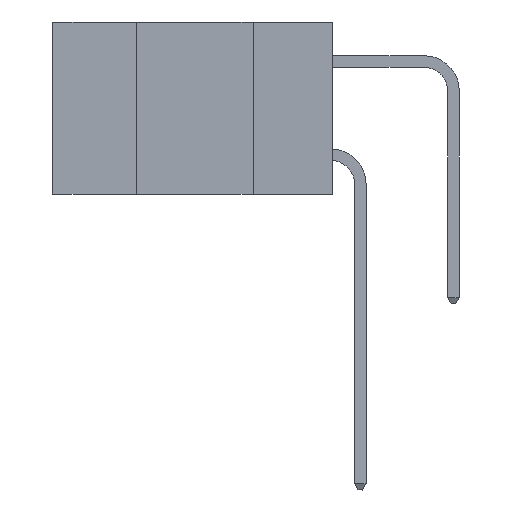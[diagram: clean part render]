
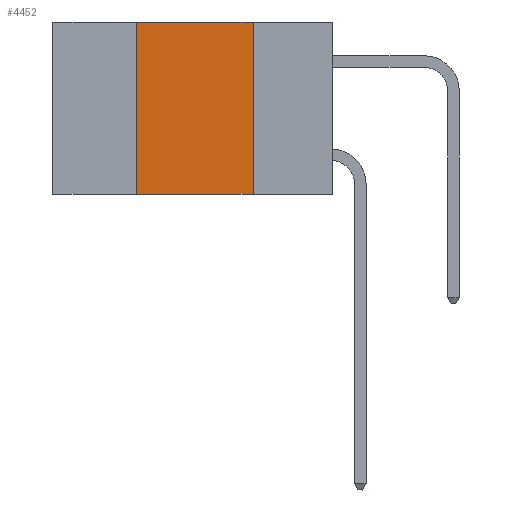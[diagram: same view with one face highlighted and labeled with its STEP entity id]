
A CAD part, left-side view. The second image highlights one B-rep face of the part: STEP entity #4452.
In plain terms, the highlighted planar face has unit normal (-1, 0, 0).
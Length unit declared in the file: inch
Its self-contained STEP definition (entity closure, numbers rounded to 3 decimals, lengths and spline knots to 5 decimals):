
#613 = ORIENTED_EDGE ( 'NONE', *, *, #7408, .F. ) ;
#865 = EDGE_CURVE ( 'NONE', #3802, #6660, #3411, .T. ) ;
#1081 = CARTESIAN_POINT ( 'NONE',  ( 0., 0.17, 0. ) ) ;
#1353 = EDGE_CURVE ( 'NONE', #3802, #3202, #12285, .T. ) ;
#3123 = CARTESIAN_POINT ( 'NONE',  ( 0., 0.17, 0. ) ) ;
#3202 = VERTEX_POINT ( 'NONE', #10478 ) ;
#3292 = DIRECTION ( 'NONE',  ( 0., 0., -1. ) ) ;
#3313 = CARTESIAN_POINT ( 'NONE',  ( 0., 0.42, -0.37 ) ) ;
#3347 = LINE ( 'NONE', #3123, #8274 ) ;
#3411 = LINE ( 'NONE', #4170, #5818 ) ;
#3802 = VERTEX_POINT ( 'NONE', #3313 ) ;
#3940 = EDGE_LOOP ( 'NONE', ( #7589, #613, #5367, #10637 ) ) ;
#4170 = CARTESIAN_POINT ( 'NONE',  ( 0., 0.42, 0. ) ) ;
#4452 = ADVANCED_FACE ( 'NONE', ( #8810 ), #8190, .F. ) ;
#4795 = CARTESIAN_POINT ( 'NONE',  ( 0., 0.6, 0. ) ) ;
#5168 = VECTOR ( 'NONE', #8775, 39.37008 ) ;
#5326 = CARTESIAN_POINT ( 'NONE',  ( 0., 0.6, 0. ) ) ;
#5367 = ORIENTED_EDGE ( 'NONE', *, *, #865, .F. ) ;
#5818 = VECTOR ( 'NONE', #9467, 39.37008 ) ;
#6283 = VECTOR ( 'NONE', #10449, 39.37008 ) ;
#6487 = CARTESIAN_POINT ( 'NONE',  ( 0., 0.6, -0.37 ) ) ;
#6660 = VERTEX_POINT ( 'NONE', #7673 ) ;
#6914 = VERTEX_POINT ( 'NONE', #1081 ) ;
#7408 = EDGE_CURVE ( 'NONE', #6660, #6914, #8781, .T. ) ;
#7589 = ORIENTED_EDGE ( 'NONE', *, *, #9722, .F. ) ;
#7673 = CARTESIAN_POINT ( 'NONE',  ( 0., 0.42, 0. ) ) ;
#8190 = PLANE ( 'NONE',  #11298 ) ;
#8274 = VECTOR ( 'NONE', #10811, 39.37008 ) ;
#8775 = DIRECTION ( 'NONE',  ( 0., -1., 0. ) ) ;
#8781 = LINE ( 'NONE', #4795, #6283 ) ;
#8810 = FACE_OUTER_BOUND ( 'NONE', #3940, .T. ) ;
#9137 = DIRECTION ( 'NONE',  ( 1., 0., 0. ) ) ;
#9467 = DIRECTION ( 'NONE',  ( 0., 0., 1. ) ) ;
#9722 = EDGE_CURVE ( 'NONE', #6914, #3202, #3347, .T. ) ;
#10449 = DIRECTION ( 'NONE',  ( 0., -1., 0. ) ) ;
#10478 = CARTESIAN_POINT ( 'NONE',  ( 0., 0.17, -0.37 ) ) ;
#10637 = ORIENTED_EDGE ( 'NONE', *, *, #1353, .T. ) ;
#10811 = DIRECTION ( 'NONE',  ( 0., 0., -1. ) ) ;
#11298 = AXIS2_PLACEMENT_3D ( 'NONE', #5326, #9137, #3292 ) ;
#12285 = LINE ( 'NONE', #6487, #5168 ) ;
